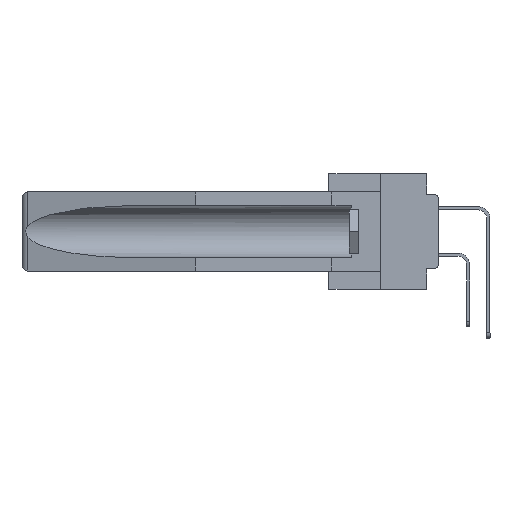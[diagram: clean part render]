
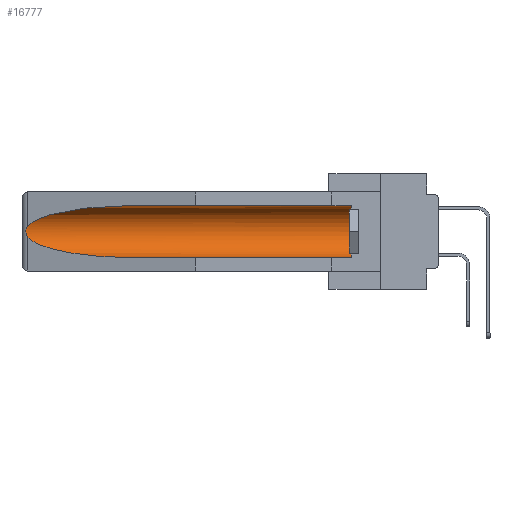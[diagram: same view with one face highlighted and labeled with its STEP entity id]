
A CAD part, left-side view. The second image highlights one B-rep face of the part: STEP entity #16777.
In plain terms, the highlighted cylindrical face has radius 2.857 mm (diameter 5.715 mm), a partial arc.
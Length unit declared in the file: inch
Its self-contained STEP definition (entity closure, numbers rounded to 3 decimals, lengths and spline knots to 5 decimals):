
#221 = VERTEX_POINT ( 'NONE', #2942 ) ;
#1404 = CARTESIAN_POINT ( 'NONE',  ( 0.2675, 1.53308, -0.17534 ) ) ;
#1810 = CARTESIAN_POINT ( 'NONE',  ( 0.26537, 1.52718, -0.14972 ) ) ;
#1885 = ORIENTED_EDGE ( 'NONE', *, *, #13281, .T. ) ;
#2291 = AXIS2_PLACEMENT_3D ( 'NONE', #3204, #27971, #34400 ) ;
#2942 = CARTESIAN_POINT ( 'NONE',  ( 0.26537, 1.52718, -0.14972 ) ) ;
#2981 = EDGE_CURVE ( 'NONE', #34717, #20610, #11044, .T. ) ;
#3204 = CARTESIAN_POINT ( 'NONE',  ( 0.155, -0.30754, -0.1715 ) ) ;
#3476 =( BOUNDED_CURVE ( )  B_SPLINE_CURVE ( 3, ( #14607, #26873, #39126, #30076 ),
 .UNSPECIFIED., .F., .F. ) 
 B_SPLINE_CURVE_WITH_KNOTS ( ( 4, 4 ),
 ( 0.1948, 1.5708 ),
 .UNSPECIFIED. ) 
 CURVE ( )  GEOMETRIC_REPRESENTATION_ITEM ( )  RATIONAL_B_SPLINE_CURVE ( ( 1., 0.848, 0.848, 1. ) ) 
 REPRESENTATION_ITEM ( '' )  );
#4515 = CARTESIAN_POINT ( 'NONE',  ( 0.155, -0.30754, -0.284 ) ) ;
#5030 = CARTESIAN_POINT ( 'NONE',  ( 0.2673, 1.5327, -0.16383 ) ) ;
#6042 = CYLINDRICAL_SURFACE ( 'NONE', #2291, 0.1125 ) ;
#6299 =( BOUNDED_CURVE ( )  B_SPLINE_CURVE ( 3, ( #33676, #20815, #24619, #27048 ),
 .UNSPECIFIED., .F., .T. ) 
 B_SPLINE_CURVE_WITH_KNOTS ( ( 4, 4 ),
 ( 4.71239, 6.08839 ),
 .UNSPECIFIED. ) 
 CURVE ( )  GEOMETRIC_REPRESENTATION_ITEM ( )  RATIONAL_B_SPLINE_CURVE ( ( 1., 0.848, 0.848, 1. ) ) 
 REPRESENTATION_ITEM ( '' )  );
#10858 = EDGE_CURVE ( 'NONE', #35638, #221, #6299, .T. ) ;
#11044 = CIRCLE ( 'NONE', #26507, 0.1125 ) ;
#11851 = EDGE_CURVE ( 'NONE', #34717, #31579, #32091, .T. ) ;
#12005 = ORIENTED_EDGE ( 'NONE', *, *, #32184, .T. ) ;
#12808 = EDGE_CURVE ( 'NONE', #221, #14968, #17214, .T. ) ;
#12956 = CARTESIAN_POINT ( 'NONE',  ( 0.155, 0.126, -0.1715 ) ) ;
#13281 = EDGE_CURVE ( 'NONE', #14968, #31579, #3476, .T. ) ;
#14173 = CARTESIAN_POINT ( 'NONE',  ( 0.155, -0.30754, -0.059 ) ) ;
#14487 = EDGE_LOOP ( 'NONE', ( #34141, #31043, #1885, #28619, #16175, #12005 ) ) ;
#14607 = CARTESIAN_POINT ( 'NONE',  ( 0.26537, 1.52718, -0.19328 ) ) ;
#14968 = VERTEX_POINT ( 'NONE', #18761 ) ;
#15791 = DIRECTION ( 'NONE',  ( 0., -1., 0. ) ) ;
#16175 = ORIENTED_EDGE ( 'NONE', *, *, #2981, .T. ) ;
#16777 = ADVANCED_FACE ( 'NONE', ( #27767 ), #6042, .F. ) ;
#16813 = DIRECTION ( 'NONE',  ( 0., 1., 0. ) ) ;
#17123 = CARTESIAN_POINT ( 'NONE',  ( 0.26597, 1.5296, -0.19026 ) ) ;
#17214 = B_SPLINE_CURVE_WITH_KNOTS ( 'NONE', 3,
 ( #1810, #38619, #38015, #5030, #29179, #1404, #23143, #31998, #17123, #22942 ),
 .UNSPECIFIED., .F., .F.,
 ( 4, 2, 2, 2, 4 ),
 ( 0., 0.00029, 0.00058, 0.00087, 0.00117 ),
 .UNSPECIFIED. ) ;
#18659 = CARTESIAN_POINT ( 'NONE',  ( 0.155, 1.07973, -0.284 ) ) ;
#18761 = CARTESIAN_POINT ( 'NONE',  ( 0.26537, 1.52718, -0.19328 ) ) ;
#20610 = VERTEX_POINT ( 'NONE', #25570 ) ;
#20815 = CARTESIAN_POINT ( 'NONE',  ( 0.21114, 1.30732, -0.059 ) ) ;
#22942 = CARTESIAN_POINT ( 'NONE',  ( 0.26537, 1.52718, -0.19328 ) ) ;
#23143 = CARTESIAN_POINT ( 'NONE',  ( 0.2673, 1.53269, -0.17917 ) ) ;
#24619 = CARTESIAN_POINT ( 'NONE',  ( 0.25451, 1.48313, -0.09465 ) ) ;
#25570 = CARTESIAN_POINT ( 'NONE',  ( 0.155, 0.126, -0.059 ) ) ;
#26507 = AXIS2_PLACEMENT_3D ( 'NONE', #12956, #15791, #34865 ) ;
#26873 = CARTESIAN_POINT ( 'NONE',  ( 0.25451, 1.48313, -0.24835 ) ) ;
#27048 = CARTESIAN_POINT ( 'NONE',  ( 0.26537, 1.52718, -0.14972 ) ) ;
#27767 = FACE_OUTER_BOUND ( 'NONE', #14487, .T. ) ;
#27971 = DIRECTION ( 'NONE',  ( 0., 1., 0. ) ) ;
#28619 = ORIENTED_EDGE ( 'NONE', *, *, #11851, .F. ) ;
#29031 = VECTOR ( 'NONE', #16813, 39.37008 ) ;
#29056 = DIRECTION ( 'NONE',  ( 0., 1., 0. ) ) ;
#29179 = CARTESIAN_POINT ( 'NONE',  ( 0.2675, 1.53308, -0.16763 ) ) ;
#29333 = VECTOR ( 'NONE', #29056, 39.37008 ) ;
#30076 = CARTESIAN_POINT ( 'NONE',  ( 0.155, 1.07973, -0.284 ) ) ;
#30116 = CARTESIAN_POINT ( 'NONE',  ( 0.155, 1.07973, -0.059 ) ) ;
#31043 = ORIENTED_EDGE ( 'NONE', *, *, #12808, .T. ) ;
#31579 = VERTEX_POINT ( 'NONE', #18659 ) ;
#31866 = LINE ( 'NONE', #14173, #29333 ) ;
#31998 = CARTESIAN_POINT ( 'NONE',  ( 0.26655, 1.53094, -0.18657 ) ) ;
#32091 = LINE ( 'NONE', #4515, #29031 ) ;
#32184 = EDGE_CURVE ( 'NONE', #20610, #35638, #31866, .T. ) ;
#33676 = CARTESIAN_POINT ( 'NONE',  ( 0.155, 1.07973, -0.059 ) ) ;
#34141 = ORIENTED_EDGE ( 'NONE', *, *, #10858, .T. ) ;
#34400 = DIRECTION ( 'NONE',  ( 0., 0., 1. ) ) ;
#34557 = CARTESIAN_POINT ( 'NONE',  ( 0.155, 0.126, -0.284 ) ) ;
#34717 = VERTEX_POINT ( 'NONE', #34557 ) ;
#34865 = DIRECTION ( 'NONE',  ( 0., 0., 1. ) ) ;
#35638 = VERTEX_POINT ( 'NONE', #30116 ) ;
#38015 = CARTESIAN_POINT ( 'NONE',  ( 0.26654, 1.53092, -0.15636 ) ) ;
#38619 = CARTESIAN_POINT ( 'NONE',  ( 0.26597, 1.52961, -0.15275 ) ) ;
#39126 = CARTESIAN_POINT ( 'NONE',  ( 0.21114, 1.30732, -0.284 ) ) ;
